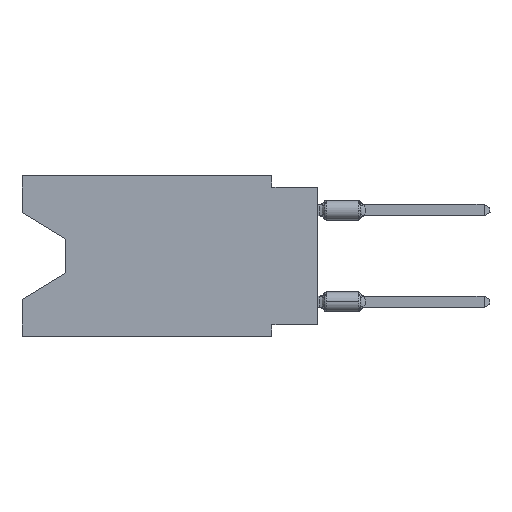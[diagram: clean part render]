
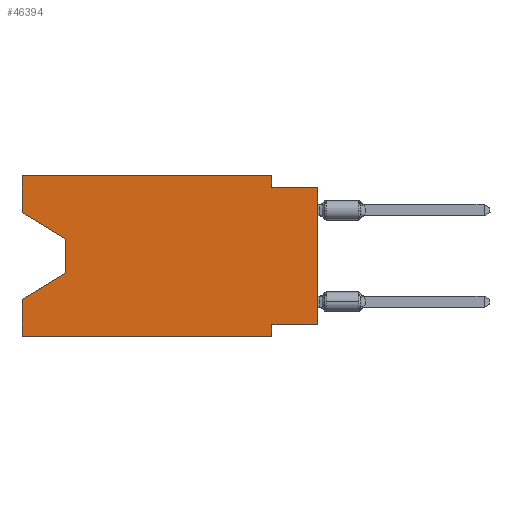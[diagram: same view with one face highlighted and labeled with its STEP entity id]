
A CAD part, left-side view. The second image highlights one B-rep face of the part: STEP entity #46394.
In plain terms, the highlighted planar face has unit normal (-1, 0, 0).
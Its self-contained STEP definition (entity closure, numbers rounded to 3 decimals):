
#258 = CARTESIAN_POINT ( 'NONE',  ( 0., 2.54, -8.89 ) ) ;
#305 = LINE ( 'NONE', #25013, #48113 ) ;
#499 = ORIENTED_EDGE ( 'NONE', *, *, #17350, .T. ) ;
#506 = ORIENTED_EDGE ( 'NONE', *, *, #19533, .T. ) ;
#666 = LINE ( 'NONE', #258, #18891 ) ;
#712 = EDGE_CURVE ( 'NONE', #11141, #35753, #24090, .T. ) ;
#1317 = VERTEX_POINT ( 'NONE', #44544 ) ;
#2275 = DIRECTION ( 'NONE',  ( 0., 0., -1. ) ) ;
#2851 = CARTESIAN_POINT ( 'NONE',  ( 0., 2.54, 0. ) ) ;
#2963 = LINE ( 'NONE', #11101, #16672 ) ;
#4816 = CARTESIAN_POINT ( 'NONE',  ( 0., 16.383, -8.89 ) ) ;
#5343 = CARTESIAN_POINT ( 'NONE',  ( 0., 16.383, 0. ) ) ;
#5415 = VECTOR ( 'NONE', #53133, 1000. ) ;
#5472 = CARTESIAN_POINT ( 'NONE',  ( 0., 2.54, -8.255 ) ) ;
#6110 = DIRECTION ( 'NONE',  ( 0., 0., -1. ) ) ;
#6189 = DIRECTION ( 'NONE',  ( 0., 0., 1. ) ) ;
#7207 = ORIENTED_EDGE ( 'NONE', *, *, #30082, .F. ) ;
#8022 = EDGE_CURVE ( 'NONE', #24920, #14612, #51758, .T. ) ;
#8713 = VECTOR ( 'NONE', #6189, 1000. ) ;
#10731 = LINE ( 'NONE', #31378, #19683 ) ;
#10942 = PLANE ( 'NONE',  #27588 ) ;
#11093 = CARTESIAN_POINT ( 'NONE',  ( 0., 0., -8.255 ) ) ;
#11101 = CARTESIAN_POINT ( 'NONE',  ( 0., 16.383, 0. ) ) ;
#11141 = VERTEX_POINT ( 'NONE', #11093 ) ;
#11798 = EDGE_LOOP ( 'NONE', ( #506, #34519, #499, #50263, #36531, #46738, #7207, #37089, #28616, #41970, #31006, #23381 ) ) ;
#12488 = EDGE_CURVE ( 'NONE', #43430, #50101, #13818, .T. ) ;
#13818 = LINE ( 'NONE', #51060, #22106 ) ;
#14503 = CARTESIAN_POINT ( 'NONE',  ( 0., 16.383, 0. ) ) ;
#14612 = VERTEX_POINT ( 'NONE', #34071 ) ;
#15051 = CARTESIAN_POINT ( 'NONE',  ( 0., 13.97, -3.505 ) ) ;
#15474 = VECTOR ( 'NONE', #6110, 1000. ) ;
#16672 = VECTOR ( 'NONE', #19527, 1000. ) ;
#17350 = EDGE_CURVE ( 'NONE', #14612, #47827, #26619, .T. ) ;
#18365 = EDGE_CURVE ( 'NONE', #1317, #35753, #45241, .T. ) ;
#18538 = CARTESIAN_POINT ( 'NONE',  ( 0., 16.383, -2.038 ) ) ;
#18891 = VECTOR ( 'NONE', #25477, 1000. ) ;
#19011 = VECTOR ( 'NONE', #23491, 1000. ) ;
#19527 = DIRECTION ( 'NONE',  ( 0., -1., 0. ) ) ;
#19533 = EDGE_CURVE ( 'NONE', #26220, #24920, #10731, .T. ) ;
#19683 = VECTOR ( 'NONE', #35989, 1000. ) ;
#22106 = VECTOR ( 'NONE', #46987, 1000. ) ;
#22347 = CARTESIAN_POINT ( 'NONE',  ( 0., 13.97, -3.505 ) ) ;
#23381 = ORIENTED_EDGE ( 'NONE', *, *, #39697, .F. ) ;
#23491 = DIRECTION ( 'NONE',  ( 0., 0., -1. ) ) ;
#24090 = LINE ( 'NONE', #49900, #49850 ) ;
#24920 = VERTEX_POINT ( 'NONE', #22347 ) ;
#25013 = CARTESIAN_POINT ( 'NONE',  ( 0., 0., -8.255 ) ) ;
#25477 = DIRECTION ( 'NONE',  ( 0., 0., -1. ) ) ;
#26220 = VERTEX_POINT ( 'NONE', #18538 ) ;
#26619 = LINE ( 'NONE', #42700, #47954 ) ;
#26838 = EDGE_CURVE ( 'NONE', #48316, #50101, #666, .T. ) ;
#27588 = AXIS2_PLACEMENT_3D ( 'NONE', #14503, #48193, #2275 ) ;
#27837 = CARTESIAN_POINT ( 'NONE',  ( 0., 0., -0.635 ) ) ;
#28140 = DIRECTION ( 'NONE',  ( 0., 0., 1. ) ) ;
#28616 = ORIENTED_EDGE ( 'NONE', *, *, #18365, .F. ) ;
#28628 = LINE ( 'NONE', #44664, #19011 ) ;
#30082 = EDGE_CURVE ( 'NONE', #11141, #48316, #305, .T. ) ;
#30360 = VECTOR ( 'NONE', #42849, 1000. ) ;
#30470 = EDGE_CURVE ( 'NONE', #45107, #38976, #2963, .T. ) ;
#31006 = ORIENTED_EDGE ( 'NONE', *, *, #30470, .F. ) ;
#31378 = CARTESIAN_POINT ( 'NONE',  ( 0., 16.383, -2.038 ) ) ;
#32572 = EDGE_CURVE ( 'NONE', #38976, #1317, #28628, .T. ) ;
#34071 = CARTESIAN_POINT ( 'NONE',  ( 0., 13.97, -5.385 ) ) ;
#34519 = ORIENTED_EDGE ( 'NONE', *, *, #8022, .T. ) ;
#34675 = LINE ( 'NONE', #5343, #30360 ) ;
#35753 = VERTEX_POINT ( 'NONE', #41706 ) ;
#35816 = CARTESIAN_POINT ( 'NONE',  ( 0., 2.54, -8.89 ) ) ;
#35989 = DIRECTION ( 'NONE',  ( 0., -0.855, -0.519 ) ) ;
#36531 = ORIENTED_EDGE ( 'NONE', *, *, #12488, .T. ) ;
#37089 = ORIENTED_EDGE ( 'NONE', *, *, #712, .T. ) ;
#38537 = LINE ( 'NONE', #51845, #8713 ) ;
#38976 = VERTEX_POINT ( 'NONE', #2851 ) ;
#39697 = EDGE_CURVE ( 'NONE', #26220, #45107, #38537, .T. ) ;
#41069 = DIRECTION ( 'NONE',  ( 0., 1., 0. ) ) ;
#41706 = CARTESIAN_POINT ( 'NONE',  ( 0., 0., -0.635 ) ) ;
#41970 = ORIENTED_EDGE ( 'NONE', *, *, #32572, .F. ) ;
#42700 = CARTESIAN_POINT ( 'NONE',  ( 0., 13.97, -5.385 ) ) ;
#42849 = DIRECTION ( 'NONE',  ( 0., 0., 1. ) ) ;
#43049 = CARTESIAN_POINT ( 'NONE',  ( 0., 16.383, 0. ) ) ;
#43430 = VERTEX_POINT ( 'NONE', #4816 ) ;
#44117 = FACE_OUTER_BOUND ( 'NONE', #11798, .T. ) ;
#44544 = CARTESIAN_POINT ( 'NONE',  ( 0., 2.54, -0.635 ) ) ;
#44597 = EDGE_CURVE ( 'NONE', #43430, #47827, #34675, .T. ) ;
#44664 = CARTESIAN_POINT ( 'NONE',  ( 0., 2.54, 0. ) ) ;
#45107 = VERTEX_POINT ( 'NONE', #43049 ) ;
#45241 = LINE ( 'NONE', #27837, #5415 ) ;
#46394 = ADVANCED_FACE ( 'NONE', ( #44117 ), #10942, .F. ) ;
#46738 = ORIENTED_EDGE ( 'NONE', *, *, #26838, .F. ) ;
#46987 = DIRECTION ( 'NONE',  ( 0., -1., 0. ) ) ;
#47827 = VERTEX_POINT ( 'NONE', #53474 ) ;
#47954 = VECTOR ( 'NONE', #51114, 1000. ) ;
#48113 = VECTOR ( 'NONE', #41069, 1000. ) ;
#48193 = DIRECTION ( 'NONE',  ( 1., 0., 0. ) ) ;
#48316 = VERTEX_POINT ( 'NONE', #5472 ) ;
#49850 = VECTOR ( 'NONE', #28140, 1000. ) ;
#49900 = CARTESIAN_POINT ( 'NONE',  ( 0., 0., 0. ) ) ;
#50101 = VERTEX_POINT ( 'NONE', #35816 ) ;
#50263 = ORIENTED_EDGE ( 'NONE', *, *, #44597, .F. ) ;
#51060 = CARTESIAN_POINT ( 'NONE',  ( 0., 16.383, -8.89 ) ) ;
#51114 = DIRECTION ( 'NONE',  ( 0., 0.855, -0.519 ) ) ;
#51758 = LINE ( 'NONE', #15051, #15474 ) ;
#51845 = CARTESIAN_POINT ( 'NONE',  ( 0., 16.383, 0. ) ) ;
#53133 = DIRECTION ( 'NONE',  ( 0., -1., 0. ) ) ;
#53474 = CARTESIAN_POINT ( 'NONE',  ( 0., 16.383, -6.852 ) ) ;
